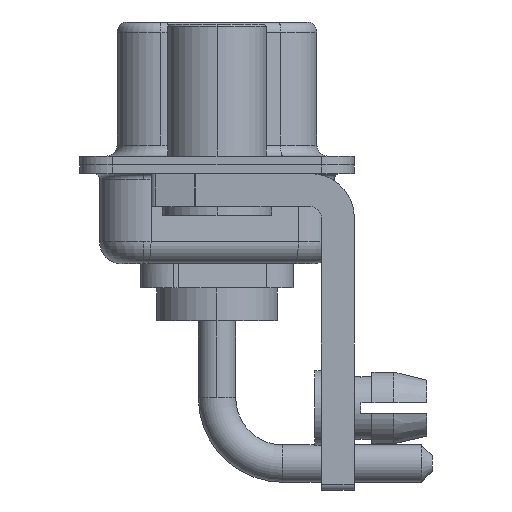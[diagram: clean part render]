
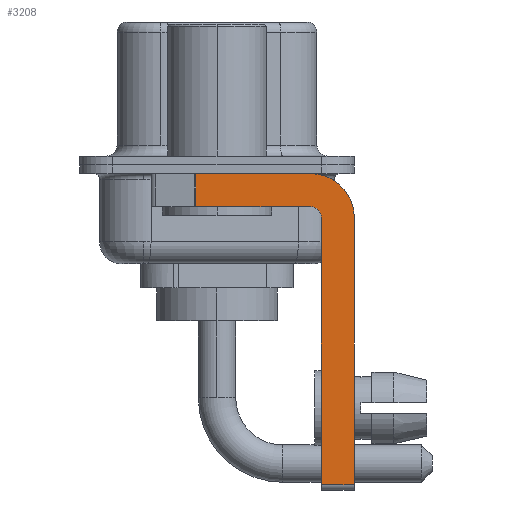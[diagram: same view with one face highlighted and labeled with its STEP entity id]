
A CAD part, left-side view. The second image highlights one B-rep face of the part: STEP entity #3208.
In plain terms, the highlighted planar face has unit normal (-1, 0, 0).
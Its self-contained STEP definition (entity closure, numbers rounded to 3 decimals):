
#292 = VECTOR ( 'NONE', #1319, 1000. ) ;
#788 = EDGE_CURVE ( 'NONE', #3466, #10300, #8162, .T. ) ;
#818 = VECTOR ( 'NONE', #16184, 1000. ) ;
#1319 = DIRECTION ( 'NONE',  ( 0., 0., 1. ) ) ;
#1335 = EDGE_CURVE ( 'NONE', #4653, #3476, #17972, .T. ) ;
#1462 = VECTOR ( 'NONE', #16973, 1000. ) ;
#2797 = EDGE_CURVE ( 'NONE', #3476, #18998, #7855, .T. ) ;
#3158 = CARTESIAN_POINT ( 'NONE',  ( -2.9, -6.25, -2.4 ) ) ;
#3208 = ADVANCED_FACE ( 'NONE', ( #4563 ), #14069, .F. ) ;
#3453 = CARTESIAN_POINT ( 'NONE',  ( -2.9, -6.25, -14.55 ) ) ;
#3466 = VERTEX_POINT ( 'NONE', #7587 ) ;
#3476 = VERTEX_POINT ( 'NONE', #7685 ) ;
#3513 = EDGE_LOOP ( 'NONE', ( #6731, #12700, #14511, #13598, #9874, #6392, #6108, #12713 ) ) ;
#3857 = EDGE_CURVE ( 'NONE', #10300, #9059, #12074, .T. ) ;
#3979 = CARTESIAN_POINT ( 'NONE',  ( -2.9, -4.25, -14.55 ) ) ;
#4190 = CARTESIAN_POINT ( 'NONE',  ( -2.9, -6.25, -2.4 ) ) ;
#4196 = CARTESIAN_POINT ( 'NONE',  ( -2.9, -4.75, -2.4 ) ) ;
#4384 = VERTEX_POINT ( 'NONE', #17498 ) ;
#4563 = FACE_OUTER_BOUND ( 'NONE', #3513, .T. ) ;
#4585 = CARTESIAN_POINT ( 'NONE',  ( -2.9, -4.25, -2.4 ) ) ;
#4653 = VERTEX_POINT ( 'NONE', #4196 ) ;
#5081 = CARTESIAN_POINT ( 'NONE',  ( -2.9, -4.75, -14.55 ) ) ;
#5132 = DIRECTION ( 'NONE',  ( 0., -1., 0. ) ) ;
#5771 = DIRECTION ( 'NONE',  ( 1., 0., 0. ) ) ;
#5983 = DIRECTION ( 'NONE',  ( 0., 0., -1. ) ) ;
#6108 = ORIENTED_EDGE ( 'NONE', *, *, #3857, .F. ) ;
#6235 = DIRECTION ( 'NONE',  ( 0., 0., -1. ) ) ;
#6392 = ORIENTED_EDGE ( 'NONE', *, *, #10134, .T. ) ;
#6533 = EDGE_CURVE ( 'NONE', #4384, #3466, #12320, .T. ) ;
#6614 = VECTOR ( 'NONE', #5132, 1000. ) ;
#6731 = ORIENTED_EDGE ( 'NONE', *, *, #6533, .F. ) ;
#7405 = EDGE_CURVE ( 'NONE', #4384, #18998, #18591, .T. ) ;
#7587 = CARTESIAN_POINT ( 'NONE',  ( -2.9, -4.25, -0.4 ) ) ;
#7685 = CARTESIAN_POINT ( 'NONE',  ( -2.9, -4.25, -1.9 ) ) ;
#7855 = LINE ( 'NONE', #9388, #9572 ) ;
#8162 = CIRCLE ( 'NONE', #18606, 2. ) ;
#8411 = CARTESIAN_POINT ( 'NONE',  ( -2.9, -4.25, -2.4 ) ) ;
#9059 = VERTEX_POINT ( 'NONE', #3453 ) ;
#9365 = CARTESIAN_POINT ( 'NONE',  ( -2.9, -4.25, -2.4 ) ) ;
#9388 = CARTESIAN_POINT ( 'NONE',  ( -2.9, -4.25, -1.9 ) ) ;
#9450 = CARTESIAN_POINT ( 'NONE',  ( -2.9, 3., -0.4 ) ) ;
#9572 = VECTOR ( 'NONE', #15628, 1000. ) ;
#9874 = ORIENTED_EDGE ( 'NONE', *, *, #19947, .F. ) ;
#10134 = EDGE_CURVE ( 'NONE', #12542, #9059, #16676, .T. ) ;
#10300 = VERTEX_POINT ( 'NONE', #3158 ) ;
#10438 = LINE ( 'NONE', #16675, #292 ) ;
#10727 = DIRECTION ( 'NONE',  ( 0., 0., 1. ) ) ;
#12074 = LINE ( 'NONE', #4190, #818 ) ;
#12320 = LINE ( 'NONE', #9450, #17301 ) ;
#12542 = VERTEX_POINT ( 'NONE', #5081 ) ;
#12587 = DIRECTION ( 'NONE',  ( 1., 0., 0. ) ) ;
#12700 = ORIENTED_EDGE ( 'NONE', *, *, #7405, .T. ) ;
#12713 = ORIENTED_EDGE ( 'NONE', *, *, #788, .F. ) ;
#13598 = ORIENTED_EDGE ( 'NONE', *, *, #1335, .F. ) ;
#13699 = CARTESIAN_POINT ( 'NONE',  ( -2.9, 0.978, -1.9 ) ) ;
#14069 = PLANE ( 'NONE',  #17767 ) ;
#14511 = ORIENTED_EDGE ( 'NONE', *, *, #2797, .F. ) ;
#15627 = DIRECTION ( 'NONE',  ( -1., 0., 0. ) ) ;
#15628 = DIRECTION ( 'NONE',  ( 0., 1., 0. ) ) ;
#16033 = AXIS2_PLACEMENT_3D ( 'NONE', #4585, #15627, #10727 ) ;
#16184 = DIRECTION ( 'NONE',  ( 0., 0., -1. ) ) ;
#16675 = CARTESIAN_POINT ( 'NONE',  ( -2.9, -4.75, -14.8 ) ) ;
#16676 = LINE ( 'NONE', #3979, #6614 ) ;
#16973 = DIRECTION ( 'NONE',  ( 0., 0., -1. ) ) ;
#17301 = VECTOR ( 'NONE', #18535, 1000. ) ;
#17498 = CARTESIAN_POINT ( 'NONE',  ( -2.9, 0.978, -0.4 ) ) ;
#17767 = AXIS2_PLACEMENT_3D ( 'NONE', #9365, #5771, #5983 ) ;
#17972 = CIRCLE ( 'NONE', #16033, 0.5 ) ;
#18357 = CARTESIAN_POINT ( 'NONE',  ( -2.9, 0.978, -1.9 ) ) ;
#18535 = DIRECTION ( 'NONE',  ( 0., -1., 0. ) ) ;
#18591 = LINE ( 'NONE', #13699, #1462 ) ;
#18606 = AXIS2_PLACEMENT_3D ( 'NONE', #8411, #12587, #6235 ) ;
#18998 = VERTEX_POINT ( 'NONE', #18357 ) ;
#19947 = EDGE_CURVE ( 'NONE', #12542, #4653, #10438, .T. ) ;
